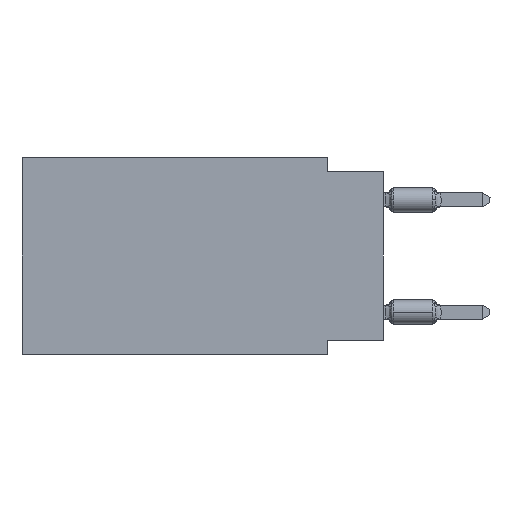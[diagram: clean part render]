
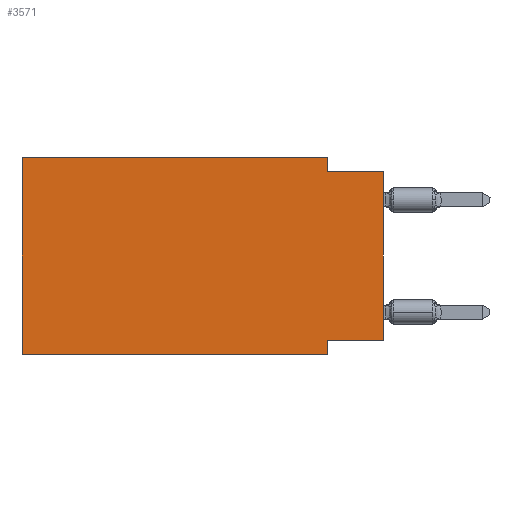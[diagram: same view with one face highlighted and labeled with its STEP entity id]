
A CAD part, left-side view. The second image highlights one B-rep face of the part: STEP entity #3571.
In plain terms, the highlighted planar face has unit normal (-1, 0, 0).
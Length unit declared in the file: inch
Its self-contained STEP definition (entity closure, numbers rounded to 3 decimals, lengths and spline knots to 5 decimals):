
#350 = LINE ( 'NONE', #19046, #7728 ) ;
#1406 = VECTOR ( 'NONE', #19473, 39.37008 ) ;
#1864 = DIRECTION ( 'NONE',  ( 0., -1., 0. ) ) ;
#2716 = CARTESIAN_POINT ( 'NONE',  ( 0., 0.1, -0.35 ) ) ;
#3571 = ADVANCED_FACE ( 'NONE', ( #54688 ), #35969, .F. ) ;
#6608 = LINE ( 'NONE', #60089, #22242 ) ;
#6678 = LINE ( 'NONE', #29547, #52602 ) ;
#7132 = DIRECTION ( 'NONE',  ( 0., 1., 0. ) ) ;
#7480 = DIRECTION ( 'NONE',  ( 0., 0., -1. ) ) ;
#7728 = VECTOR ( 'NONE', #57689, 39.37008 ) ;
#8868 = DIRECTION ( 'NONE',  ( 0., -1., 0. ) ) ;
#9779 = ORIENTED_EDGE ( 'NONE', *, *, #51281, .F. ) ;
#10803 = CARTESIAN_POINT ( 'NONE',  ( 0., 0.645, 0. ) ) ;
#11090 = VERTEX_POINT ( 'NONE', #2716 ) ;
#11856 = CARTESIAN_POINT ( 'NONE',  ( 0., 0.1, -0.325 ) ) ;
#12309 = VERTEX_POINT ( 'NONE', #50651 ) ;
#12630 = CARTESIAN_POINT ( 'NONE',  ( 0., 0.1, 0. ) ) ;
#14407 = CARTESIAN_POINT ( 'NONE',  ( 0., 0.645, 0. ) ) ;
#15875 = DIRECTION ( 'NONE',  ( 0., 0., -1. ) ) ;
#16977 = DIRECTION ( 'NONE',  ( 1., 0., 0. ) ) ;
#17669 = DIRECTION ( 'NONE',  ( 0., 0., 1. ) ) ;
#18031 = VERTEX_POINT ( 'NONE', #12630 ) ;
#18851 = VERTEX_POINT ( 'NONE', #27359 ) ;
#19046 = CARTESIAN_POINT ( 'NONE',  ( 0., 0.1, -0.35 ) ) ;
#19473 = DIRECTION ( 'NONE',  ( 0., -1., 0. ) ) ;
#21178 = LINE ( 'NONE', #50951, #27909 ) ;
#22242 = VECTOR ( 'NONE', #17669, 39.37008 ) ;
#22316 = CARTESIAN_POINT ( 'NONE',  ( 0., 0., -0.325 ) ) ;
#22964 = EDGE_CURVE ( 'NONE', #18031, #18851, #6678, .T. ) ;
#23535 = EDGE_CURVE ( 'NONE', #41218, #12309, #6608, .T. ) ;
#23574 = ORIENTED_EDGE ( 'NONE', *, *, #50104, .F. ) ;
#24246 = LINE ( 'NONE', #48622, #1406 ) ;
#24394 = ORIENTED_EDGE ( 'NONE', *, *, #22964, .F. ) ;
#25304 = VECTOR ( 'NONE', #8868, 39.37008 ) ;
#26763 = LINE ( 'NONE', #22316, #37145 ) ;
#27359 = CARTESIAN_POINT ( 'NONE',  ( 0., 0.1, -0.025 ) ) ;
#27909 = VECTOR ( 'NONE', #1864, 39.37008 ) ;
#29547 = CARTESIAN_POINT ( 'NONE',  ( 0., 0.1, 0. ) ) ;
#31815 = ORIENTED_EDGE ( 'NONE', *, *, #48976, .F. ) ;
#32219 = VERTEX_POINT ( 'NONE', #11856 ) ;
#34621 = CARTESIAN_POINT ( 'NONE',  ( 0., 0.645, -0.35 ) ) ;
#34667 = CARTESIAN_POINT ( 'NONE',  ( 0., 0., -0.325 ) ) ;
#35877 = ORIENTED_EDGE ( 'NONE', *, *, #40754, .F. ) ;
#35969 = PLANE ( 'NONE',  #53129 ) ;
#36531 = EDGE_CURVE ( 'NONE', #41218, #32219, #26763, .T. ) ;
#36612 = ORIENTED_EDGE ( 'NONE', *, *, #45496, .T. ) ;
#37145 = VECTOR ( 'NONE', #7132, 39.37008 ) ;
#40754 = EDGE_CURVE ( 'NONE', #41152, #18031, #42107, .T. ) ;
#41152 = VERTEX_POINT ( 'NONE', #14407 ) ;
#41218 = VERTEX_POINT ( 'NONE', #34667 ) ;
#42107 = LINE ( 'NONE', #42439, #25304 ) ;
#42155 = ORIENTED_EDGE ( 'NONE', *, *, #36531, .F. ) ;
#42439 = CARTESIAN_POINT ( 'NONE',  ( 0., 0.645, 0. ) ) ;
#44370 = DIRECTION ( 'NONE',  ( 0., 0., 1. ) ) ;
#45496 = EDGE_CURVE ( 'NONE', #49646, #11090, #24246, .T. ) ;
#48622 = CARTESIAN_POINT ( 'NONE',  ( 0., 0.645, -0.35 ) ) ;
#48949 = EDGE_LOOP ( 'NONE', ( #53580, #31815, #24394, #35877, #9779, #36612, #23574, #42155 ) ) ;
#48976 = EDGE_CURVE ( 'NONE', #18851, #12309, #21178, .T. ) ;
#49646 = VERTEX_POINT ( 'NONE', #34621 ) ;
#50104 = EDGE_CURVE ( 'NONE', #32219, #11090, #350, .T. ) ;
#50651 = CARTESIAN_POINT ( 'NONE',  ( 0., 0., -0.025 ) ) ;
#50951 = CARTESIAN_POINT ( 'NONE',  ( 0., 0., -0.025 ) ) ;
#51281 = EDGE_CURVE ( 'NONE', #49646, #41152, #52951, .T. ) ;
#52602 = VECTOR ( 'NONE', #15875, 39.37008 ) ;
#52951 = LINE ( 'NONE', #10803, #55375 ) ;
#53129 = AXIS2_PLACEMENT_3D ( 'NONE', #55624, #16977, #7480 ) ;
#53580 = ORIENTED_EDGE ( 'NONE', *, *, #23535, .T. ) ;
#54688 = FACE_OUTER_BOUND ( 'NONE', #48949, .T. ) ;
#55375 = VECTOR ( 'NONE', #44370, 39.37008 ) ;
#55624 = CARTESIAN_POINT ( 'NONE',  ( 0., 0.645, 0. ) ) ;
#57689 = DIRECTION ( 'NONE',  ( 0., 0., -1. ) ) ;
#60089 = CARTESIAN_POINT ( 'NONE',  ( 0., 0., 0. ) ) ;
